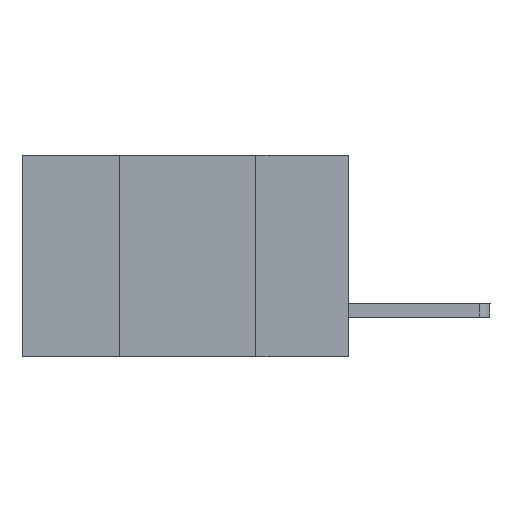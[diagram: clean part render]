
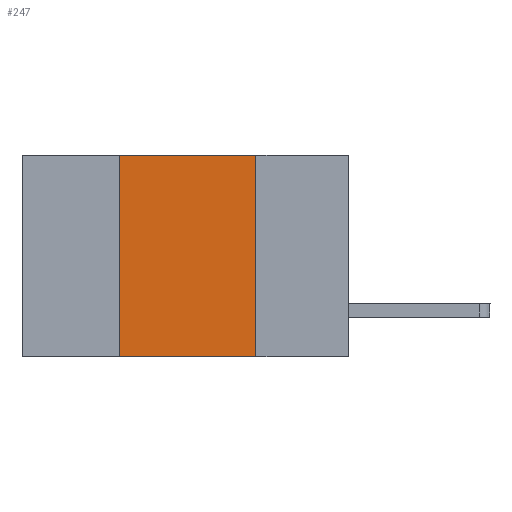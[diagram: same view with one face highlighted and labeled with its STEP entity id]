
A CAD part, left-side view. The second image highlights one B-rep face of the part: STEP entity #247.
In plain terms, the highlighted planar face has unit normal (-1, 0, 0).
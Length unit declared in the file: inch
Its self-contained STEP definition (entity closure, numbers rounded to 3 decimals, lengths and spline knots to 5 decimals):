
#17 = ORIENTED_EDGE ( 'NONE', *, *, #7710, .F. ) ;
#20 = VERTEX_POINT ( 'NONE', #4446 ) ;
#247 = ADVANCED_FACE ( 'NONE', ( #4518 ), #9381, .F. ) ;
#1773 = DIRECTION ( 'NONE',  ( 0., 0., -1. ) ) ;
#1871 = AXIS2_PLACEMENT_3D ( 'NONE', #4769, #5590, #1773 ) ;
#2278 = LINE ( 'NONE', #4805, #8078 ) ;
#2597 = VERTEX_POINT ( 'NONE', #9533 ) ;
#3256 = VECTOR ( 'NONE', #4497, 39.37008 ) ;
#3265 = EDGE_CURVE ( 'NONE', #8940, #8834, #8107, .T. ) ;
#3890 = VECTOR ( 'NONE', #6423, 39.37008 ) ;
#4272 = LINE ( 'NONE', #9093, #6532 ) ;
#4446 = CARTESIAN_POINT ( 'NONE',  ( 0., 0.17, 0. ) ) ;
#4497 = DIRECTION ( 'NONE',  ( 0., -1., 0. ) ) ;
#4518 = FACE_OUTER_BOUND ( 'NONE', #6045, .T. ) ;
#4554 = DIRECTION ( 'NONE',  ( 0., 0., 1. ) ) ;
#4769 = CARTESIAN_POINT ( 'NONE',  ( 0., 0.6, 0. ) ) ;
#4805 = CARTESIAN_POINT ( 'NONE',  ( 0., 0.6, 0. ) ) ;
#5590 = DIRECTION ( 'NONE',  ( 1., 0., 0. ) ) ;
#5947 = EDGE_CURVE ( 'NONE', #2597, #20, #2278, .T. ) ;
#6045 = EDGE_LOOP ( 'NONE', ( #7481, #8190, #17, #8521 ) ) ;
#6423 = DIRECTION ( 'NONE',  ( 0., 0., -1. ) ) ;
#6532 = VECTOR ( 'NONE', #4554, 39.37008 ) ;
#7481 = ORIENTED_EDGE ( 'NONE', *, *, #8516, .F. ) ;
#7710 = EDGE_CURVE ( 'NONE', #8940, #2597, #4272, .T. ) ;
#7856 = DIRECTION ( 'NONE',  ( 0., -1., 0. ) ) ;
#8078 = VECTOR ( 'NONE', #7856, 39.37008 ) ;
#8107 = LINE ( 'NONE', #9279, #3256 ) ;
#8159 = CARTESIAN_POINT ( 'NONE',  ( 0., 0.42, -0.37 ) ) ;
#8190 = ORIENTED_EDGE ( 'NONE', *, *, #5947, .F. ) ;
#8498 = LINE ( 'NONE', #9344, #3890 ) ;
#8516 = EDGE_CURVE ( 'NONE', #20, #8834, #8498, .T. ) ;
#8521 = ORIENTED_EDGE ( 'NONE', *, *, #3265, .T. ) ;
#8834 = VERTEX_POINT ( 'NONE', #9662 ) ;
#8940 = VERTEX_POINT ( 'NONE', #8159 ) ;
#9093 = CARTESIAN_POINT ( 'NONE',  ( 0., 0.42, 0. ) ) ;
#9279 = CARTESIAN_POINT ( 'NONE',  ( 0., 0.6, -0.37 ) ) ;
#9344 = CARTESIAN_POINT ( 'NONE',  ( 0., 0.17, 0. ) ) ;
#9381 = PLANE ( 'NONE',  #1871 ) ;
#9533 = CARTESIAN_POINT ( 'NONE',  ( 0., 0.42, 0. ) ) ;
#9662 = CARTESIAN_POINT ( 'NONE',  ( 0., 0.17, -0.37 ) ) ;
